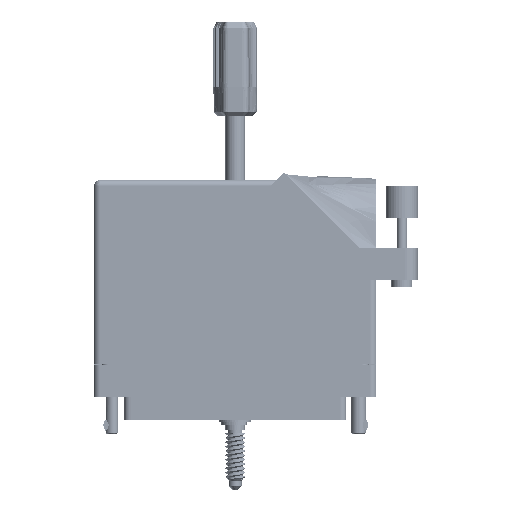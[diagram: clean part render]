
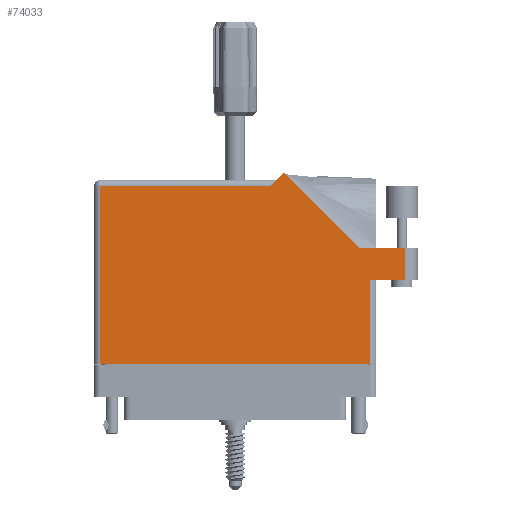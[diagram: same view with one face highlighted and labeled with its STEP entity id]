
A CAD part, front view. The second image highlights one B-rep face of the part: STEP entity #74033.
In plain terms, the highlighted face is planar.
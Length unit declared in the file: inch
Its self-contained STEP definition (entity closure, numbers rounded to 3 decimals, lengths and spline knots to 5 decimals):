
#550 = VERTEX_POINT ( 'NONE', #88486 ) ;
#639 = VERTEX_POINT ( 'NONE', #923 ) ;
#923 = CARTESIAN_POINT ( 'NONE',  ( -1.297, 1.613, 0.617 ) ) ;
#2052 = VECTOR ( 'NONE', #15857, 39.37008 ) ;
#2479 = EDGE_CURVE ( 'NONE', #75533, #30258, #62034, .T. ) ;
#3379 = ORIENTED_EDGE ( 'NONE', *, *, #60356, .T. ) ;
#3387 = VECTOR ( 'NONE', #33138, 39.37008 ) ;
#4315 = EDGE_CURVE ( 'NONE', #48137, #639, #61390, .T. ) ;
#6710 = EDGE_CURVE ( 'NONE', #30258, #54987, #10604, .T. ) ;
#7613 = AXIS2_PLACEMENT_3D ( 'NONE', #63908, #19068, #93080 ) ;
#8370 = DIRECTION ( 'NONE',  ( 0., 1., 0. ) ) ;
#8892 = EDGE_CURVE ( 'NONE', #639, #29466, #85435, .T. ) ;
#9128 = CARTESIAN_POINT ( 'NONE',  ( -1.359, -0.1, 0.617 ) ) ;
#10133 = CARTESIAN_POINT ( 'NONE',  ( -1.297, -0.1, 0.617 ) ) ;
#10379 = LINE ( 'NONE', #30394, #74873 ) ;
#10604 = LINE ( 'NONE', #16642, #63335 ) ;
#11197 = PLANE ( 'NONE',  #7613 ) ;
#12511 = LINE ( 'NONE', #9128, #88638 ) ;
#15857 = DIRECTION ( 'NONE',  ( -0.707, -0.707, 0. ) ) ;
#16642 = CARTESIAN_POINT ( 'NONE',  ( 1.19342, 1.022, 0.617 ) ) ;
#16931 = VERTEX_POINT ( 'NONE', #92115 ) ;
#17142 = VECTOR ( 'NONE', #18661, 39.37008 ) ;
#17676 = DIRECTION ( 'NONE',  ( 1., 0., 0. ) ) ;
#18396 = CARTESIAN_POINT ( 'NONE',  ( 0.337, 1.613, 0.617 ) ) ;
#18661 = DIRECTION ( 'NONE',  ( 0., 1., 0. ) ) ;
#19068 = DIRECTION ( 'NONE',  ( 0., 0., -1. ) ) ;
#19810 = ORIENTED_EDGE ( 'NONE', *, *, #8892, .T. ) ;
#23845 = ORIENTED_EDGE ( 'NONE', *, *, #50034, .T. ) ;
#27398 = ORIENTED_EDGE ( 'NONE', *, *, #6710, .T. ) ;
#29466 = VERTEX_POINT ( 'NONE', #47615 ) ;
#30216 = FACE_OUTER_BOUND ( 'NONE', #37979, .T. ) ;
#30258 = VERTEX_POINT ( 'NONE', #33332 ) ;
#30394 = CARTESIAN_POINT ( 'NONE',  ( 1.297, 0.715, 0.617 ) ) ;
#32170 = VECTOR ( 'NONE', #68886, 39.37008 ) ;
#33138 = DIRECTION ( 'NONE',  ( 0., -1., 0. ) ) ;
#33332 = CARTESIAN_POINT ( 'NONE',  ( 1.19342, 1.022, 0.617 ) ) ;
#37115 = LINE ( 'NONE', #79264, #17142 ) ;
#37979 = EDGE_LOOP ( 'NONE', ( #53119, #23845, #67361, #27398, #65283, #74237, #19810, #63562, #3379 ) ) ;
#38314 = DIRECTION ( 'NONE',  ( -0.707, 0.707, 0. ) ) ;
#45643 = VECTOR ( 'NONE', #88485, 39.37008 ) ;
#47298 = CARTESIAN_POINT ( 'NONE',  ( 1.359, 0.715, 0.617 ) ) ;
#47615 = CARTESIAN_POINT ( 'NONE',  ( -1.297, -0.1, 0.617 ) ) ;
#48137 = VERTEX_POINT ( 'NONE', #18396 ) ;
#49462 = VECTOR ( 'NONE', #76728, 39.37008 ) ;
#50034 = EDGE_CURVE ( 'NONE', #51846, #75533, #37115, .T. ) ;
#51846 = VERTEX_POINT ( 'NONE', #52659 ) ;
#52548 = EDGE_CURVE ( 'NONE', #550, #51846, #89303, .T. ) ;
#52659 = CARTESIAN_POINT ( 'NONE',  ( 1.634, 0.715, 0.617 ) ) ;
#53119 = ORIENTED_EDGE ( 'NONE', *, *, #52548, .T. ) ;
#54987 = VERTEX_POINT ( 'NONE', #73743 ) ;
#57672 = CARTESIAN_POINT ( 'NONE',  ( 1.759, 1.022, 0.617 ) ) ;
#60356 = EDGE_CURVE ( 'NONE', #16931, #550, #10379, .T. ) ;
#61390 = LINE ( 'NONE', #91172, #32170 ) ;
#62034 = LINE ( 'NONE', #57672, #45643 ) ;
#63335 = VECTOR ( 'NONE', #38314, 39.37008 ) ;
#63406 = CARTESIAN_POINT ( 'NONE',  ( 1.634, 1.022, 0.617 ) ) ;
#63562 = ORIENTED_EDGE ( 'NONE', *, *, #74383, .T. ) ;
#63908 = CARTESIAN_POINT ( 'NONE',  ( -1.359, 1.675, 0.617 ) ) ;
#65283 = ORIENTED_EDGE ( 'NONE', *, *, #81485, .T. ) ;
#67361 = ORIENTED_EDGE ( 'NONE', *, *, #2479, .T. ) ;
#68554 = CARTESIAN_POINT ( 'NONE',  ( 0.399, 1.675, 0.617 ) ) ;
#68886 = DIRECTION ( 'NONE',  ( -1., 0., 0. ) ) ;
#73743 = CARTESIAN_POINT ( 'NONE',  ( 0.46971, 1.74571, 0.617 ) ) ;
#74033 = ADVANCED_FACE ( 'NONE', ( #30216 ), #11197, .F. ) ;
#74237 = ORIENTED_EDGE ( 'NONE', *, *, #4315, .T. ) ;
#74383 = EDGE_CURVE ( 'NONE', #29466, #16931, #12511, .T. ) ;
#74873 = VECTOR ( 'NONE', #8370, 39.37008 ) ;
#75533 = VERTEX_POINT ( 'NONE', #63406 ) ;
#76728 = DIRECTION ( 'NONE',  ( 1., 0., 0. ) ) ;
#79264 = CARTESIAN_POINT ( 'NONE',  ( 1.634, 1.022, 0.617 ) ) ;
#81485 = EDGE_CURVE ( 'NONE', #54987, #48137, #82941, .T. ) ;
#82941 = LINE ( 'NONE', #68554, #2052 ) ;
#85435 = LINE ( 'NONE', #10133, #3387 ) ;
#88485 = DIRECTION ( 'NONE',  ( -1., 0., 0. ) ) ;
#88486 = CARTESIAN_POINT ( 'NONE',  ( 1.297, 0.715, 0.617 ) ) ;
#88638 = VECTOR ( 'NONE', #17676, 39.37008 ) ;
#89303 = LINE ( 'NONE', #47298, #49462 ) ;
#91172 = CARTESIAN_POINT ( 'NONE',  ( -1.359, 1.613, 0.617 ) ) ;
#92115 = CARTESIAN_POINT ( 'NONE',  ( 1.297, -0.1, 0.617 ) ) ;
#93080 = DIRECTION ( 'NONE',  ( -1., 0., 0. ) ) ;
